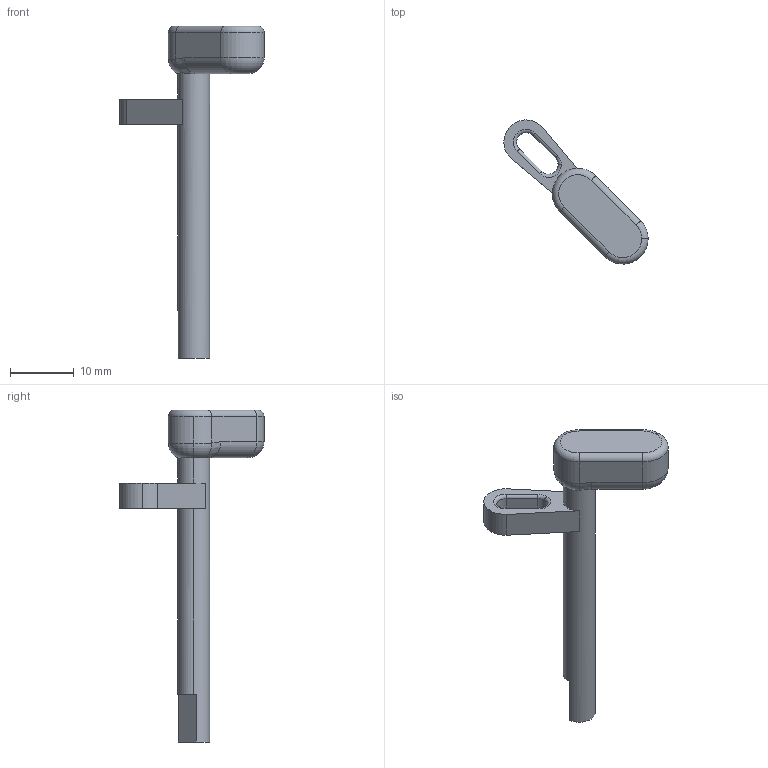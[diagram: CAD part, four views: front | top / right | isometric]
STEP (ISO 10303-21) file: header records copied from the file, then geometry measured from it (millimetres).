
FILE_DESCRIPTION (( 'STEP AP214' ), '1' );
FILE_NAME ('Mag_Release_Arm.step', '2014-05-14T06:09:24', ( 'WarFairy' ), ( '' ), 'SwSTEP 2.0', 'SolidWorks 2013', '' );
FILE_SCHEMA (( 'AUTOMOTIVE_DESIGN' ));
Length unit declared in the file: inch
Products named in the file (1): Mag_Release_Arm
Bounding box: 22.7 x 22.69 x 52.25 mm (x, y, z)
Volume: 1997.3 mm3; surface area: 1516.2 mm2
Topology: 1 solids, 1 shells, 46 faces, 112 edges, 68 vertices
Faces by surface type: cylinder 18, torus 13, plane 13, bspline 2
Entity records: 1476 total; most frequent: CARTESIAN_POINT 316, DIRECTION 262, ORIENTED_EDGE 224, EDGE_CURVE 112, AXIS2_PLACEMENT_3D 110, VERTEX_POINT 68, CIRCLE 65, EDGE_LOOP 48
